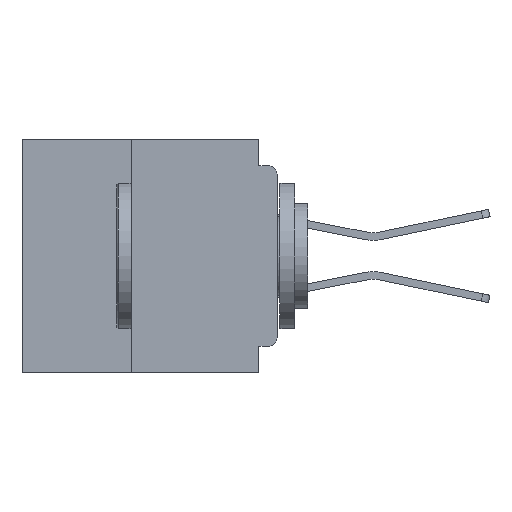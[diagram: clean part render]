
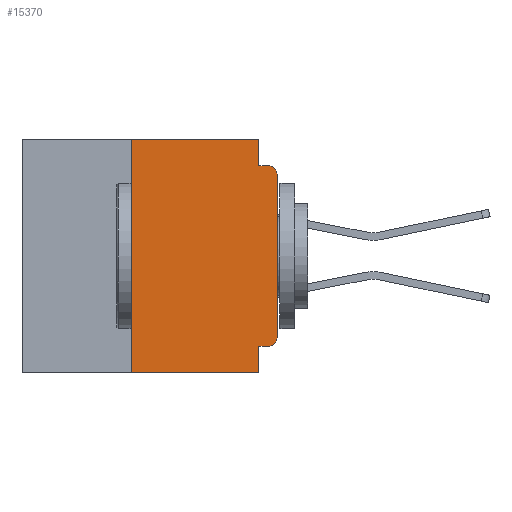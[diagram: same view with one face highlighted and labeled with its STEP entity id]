
A CAD part, left-side view. The second image highlights one B-rep face of the part: STEP entity #15370.
In plain terms, the highlighted planar face has unit normal (-1, 0, 0).
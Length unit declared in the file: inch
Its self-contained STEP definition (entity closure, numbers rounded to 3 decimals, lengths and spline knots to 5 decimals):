
#384 = CARTESIAN_POINT ( 'NONE',  ( 0., 0.25, 0. ) ) ;
#1433 = DIRECTION ( 'NONE',  ( 0., 0., -1. ) ) ;
#2754 = CARTESIAN_POINT ( 'NONE',  ( 0., 0., -0.34 ) ) ;
#4126 = LINE ( 'NONE', #21661, #33704 ) ;
#4365 = VERTEX_POINT ( 'NONE', #28155 ) ;
#4400 = DIRECTION ( 'NONE',  ( 0., 1., 0. ) ) ;
#4514 = LINE ( 'NONE', #47574, #46014 ) ;
#4622 = EDGE_CURVE ( 'NONE', #38341, #37678, #48111, .T. ) ;
#4709 = AXIS2_PLACEMENT_3D ( 'NONE', #20460, #48520, #24522 ) ;
#5260 = LINE ( 'NONE', #30238, #44245 ) ;
#6707 = EDGE_CURVE ( 'NONE', #14969, #11946, #22884, .T. ) ;
#7274 = CARTESIAN_POINT ( 'NONE',  ( 0., 0.437, 0. ) ) ;
#8147 = ORIENTED_EDGE ( 'NONE', *, *, #25313, .F. ) ;
#8699 = LINE ( 'NONE', #39918, #40780 ) ;
#9508 = DIRECTION ( 'NONE',  ( 0., -1., 0. ) ) ;
#11946 = VERTEX_POINT ( 'NONE', #2754 ) ;
#12027 = FACE_OUTER_BOUND ( 'NONE', #40000, .T. ) ;
#13459 = ORIENTED_EDGE ( 'NONE', *, *, #46121, .F. ) ;
#13590 = ORIENTED_EDGE ( 'NONE', *, *, #37379, .F. ) ;
#13764 = ORIENTED_EDGE ( 'NONE', *, *, #4622, .F. ) ;
#14963 = LINE ( 'NONE', #48978, #45773 ) ;
#14969 = VERTEX_POINT ( 'NONE', #15937 ) ;
#15197 = PLANE ( 'NONE',  #19456 ) ;
#15362 = VECTOR ( 'NONE', #4400, 39.37008 ) ;
#15370 = ADVANCED_FACE ( 'NONE', ( #12027 ), #15197, .F. ) ;
#15937 = CARTESIAN_POINT ( 'NONE',  ( 0., 0.015, -0.355 ) ) ;
#16884 = DIRECTION ( 'NONE',  ( 0., 0., 1. ) ) ;
#17395 = VECTOR ( 'NONE', #1433, 39.37008 ) ;
#17471 = CARTESIAN_POINT ( 'NONE',  ( 0., 0.031, -0.4 ) ) ;
#18333 = EDGE_CURVE ( 'NONE', #37401, #41537, #4126, .T. ) ;
#18678 = ORIENTED_EDGE ( 'NONE', *, *, #23077, .T. ) ;
#19456 = AXIS2_PLACEMENT_3D ( 'NONE', #7274, #19461, #47509 ) ;
#19461 = DIRECTION ( 'NONE',  ( 1., 0., 0. ) ) ;
#20460 = CARTESIAN_POINT ( 'NONE',  ( 0., 0.015, -0.34 ) ) ;
#20707 = ORIENTED_EDGE ( 'NONE', *, *, #37675, .T. ) ;
#21041 = CARTESIAN_POINT ( 'NONE',  ( 0., 0.031, -0.045 ) ) ;
#21661 = CARTESIAN_POINT ( 'NONE',  ( 0., 0.437, 0. ) ) ;
#22202 = CARTESIAN_POINT ( 'NONE',  ( 0., 0.015, -0.06 ) ) ;
#22884 = CIRCLE ( 'NONE', #4709, 0.015 ) ;
#23077 = EDGE_CURVE ( 'NONE', #49775, #37678, #4514, .T. ) ;
#24522 = DIRECTION ( 'NONE',  ( 0., 0., -1. ) ) ;
#24849 = EDGE_CURVE ( 'NONE', #41537, #25907, #25750, .T. ) ;
#24852 = EDGE_CURVE ( 'NONE', #4365, #41731, #47078, .T. ) ;
#25313 = EDGE_CURVE ( 'NONE', #49775, #37401, #14963, .T. ) ;
#25750 = LINE ( 'NONE', #34109, #45823 ) ;
#25907 = VERTEX_POINT ( 'NONE', #21041 ) ;
#26044 = CARTESIAN_POINT ( 'NONE',  ( 0., 0.031, -0.4 ) ) ;
#26092 = LINE ( 'NONE', #44465, #15362 ) ;
#26246 = DIRECTION ( 'NONE',  ( 0., 0., -1. ) ) ;
#26326 = CARTESIAN_POINT ( 'NONE',  ( 0., 0.031, -0.355 ) ) ;
#28155 = CARTESIAN_POINT ( 'NONE',  ( 0., 0., -0.06 ) ) ;
#30238 = CARTESIAN_POINT ( 'NONE',  ( 0., 0., 0. ) ) ;
#33704 = VECTOR ( 'NONE', #9508, 39.37008 ) ;
#34109 = CARTESIAN_POINT ( 'NONE',  ( 0., 0.031, 0. ) ) ;
#34863 = AXIS2_PLACEMENT_3D ( 'NONE', #22202, #50233, #26246 ) ;
#35626 = DIRECTION ( 'NONE',  ( 0., -1., 0. ) ) ;
#37379 = EDGE_CURVE ( 'NONE', #14969, #38341, #26092, .T. ) ;
#37401 = VERTEX_POINT ( 'NONE', #384 ) ;
#37675 = EDGE_CURVE ( 'NONE', #11946, #4365, #5260, .T. ) ;
#37678 = VERTEX_POINT ( 'NONE', #26044 ) ;
#38162 = DIRECTION ( 'NONE',  ( 0., 0., -1. ) ) ;
#38341 = VERTEX_POINT ( 'NONE', #26326 ) ;
#39918 = CARTESIAN_POINT ( 'NONE',  ( 0., 0., -0.045 ) ) ;
#40000 = EDGE_LOOP ( 'NONE', ( #20707, #49996, #13459, #40163, #46580, #8147, #18678, #13764, #13590, #49068 ) ) ;
#40163 = ORIENTED_EDGE ( 'NONE', *, *, #24849, .F. ) ;
#40780 = VECTOR ( 'NONE', #47980, 39.37008 ) ;
#41537 = VERTEX_POINT ( 'NONE', #45306 ) ;
#41731 = VERTEX_POINT ( 'NONE', #42491 ) ;
#42094 = CARTESIAN_POINT ( 'NONE',  ( 0., 0.25, -0.4 ) ) ;
#42491 = CARTESIAN_POINT ( 'NONE',  ( 0., 0.015, -0.045 ) ) ;
#44245 = VECTOR ( 'NONE', #50211, 39.37008 ) ;
#44465 = CARTESIAN_POINT ( 'NONE',  ( 0., 0., -0.355 ) ) ;
#45306 = CARTESIAN_POINT ( 'NONE',  ( 0., 0.031, 0. ) ) ;
#45773 = VECTOR ( 'NONE', #16884, 39.37008 ) ;
#45823 = VECTOR ( 'NONE', #38162, 39.37008 ) ;
#46014 = VECTOR ( 'NONE', #35626, 39.37008 ) ;
#46121 = EDGE_CURVE ( 'NONE', #25907, #41731, #8699, .T. ) ;
#46580 = ORIENTED_EDGE ( 'NONE', *, *, #18333, .F. ) ;
#47078 = CIRCLE ( 'NONE', #34863, 0.015 ) ;
#47509 = DIRECTION ( 'NONE',  ( 0., 0., -1. ) ) ;
#47574 = CARTESIAN_POINT ( 'NONE',  ( 0., 0.437, -0.4 ) ) ;
#47980 = DIRECTION ( 'NONE',  ( 0., -1., 0. ) ) ;
#48111 = LINE ( 'NONE', #17471, #17395 ) ;
#48520 = DIRECTION ( 'NONE',  ( -1., 0., 0. ) ) ;
#48978 = CARTESIAN_POINT ( 'NONE',  ( 0., 0.25, -0.4 ) ) ;
#49068 = ORIENTED_EDGE ( 'NONE', *, *, #6707, .T. ) ;
#49775 = VERTEX_POINT ( 'NONE', #42094 ) ;
#49996 = ORIENTED_EDGE ( 'NONE', *, *, #24852, .T. ) ;
#50211 = DIRECTION ( 'NONE',  ( 0., 0., 1. ) ) ;
#50233 = DIRECTION ( 'NONE',  ( -1., 0., 0. ) ) ;
